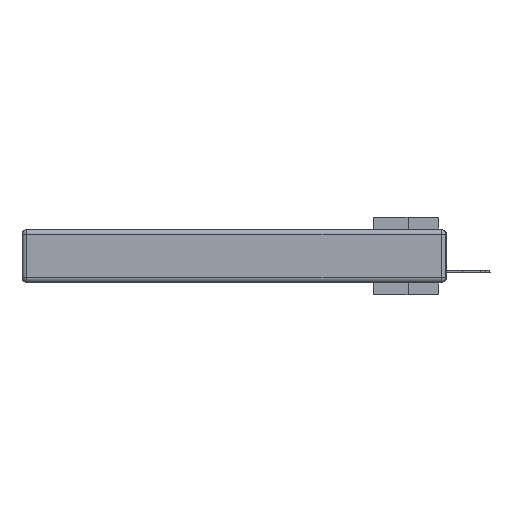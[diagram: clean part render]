
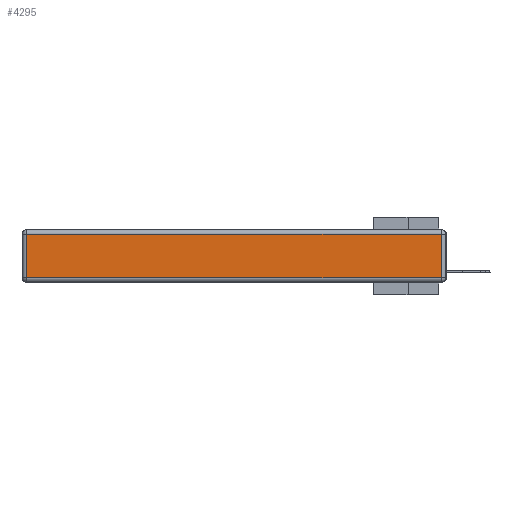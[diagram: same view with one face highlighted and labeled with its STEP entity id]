
A CAD part, left-side view. The second image highlights one B-rep face of the part: STEP entity #4295.
In plain terms, the highlighted planar face has unit normal (-1, 0, 0).
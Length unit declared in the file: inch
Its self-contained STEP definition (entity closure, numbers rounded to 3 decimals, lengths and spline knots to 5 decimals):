
#3373 = VECTOR ( 'NONE', #16008, 39.37008 ) ;
#3654 = VERTEX_POINT ( 'NONE', #3738 ) ;
#3738 = CARTESIAN_POINT ( 'NONE',  ( 0., 0.03, -0.03 ) ) ;
#4295 = ADVANCED_FACE ( 'NONE', ( #15948 ), #12384, .T. ) ;
#4736 = LINE ( 'NONE', #27565, #24641 ) ;
#5102 = ORIENTED_EDGE ( 'NONE', *, *, #26603, .T. ) ;
#5392 = CARTESIAN_POINT ( 'NONE',  ( 0., 2.72, -0.343 ) ) ;
#5779 = CARTESIAN_POINT ( 'NONE',  ( 0., 0., -0.313 ) ) ;
#5972 = DIRECTION ( 'NONE',  ( -1., 0., 0. ) ) ;
#6098 = VECTOR ( 'NONE', #14090, 39.37008 ) ;
#9346 = CARTESIAN_POINT ( 'NONE',  ( 0., 0.03, -0.313 ) ) ;
#10576 = VERTEX_POINT ( 'NONE', #12499 ) ;
#10674 = LINE ( 'NONE', #5779, #11025 ) ;
#11025 = VECTOR ( 'NONE', #21123, 39.37008 ) ;
#12384 = PLANE ( 'NONE',  #12468 ) ;
#12468 = AXIS2_PLACEMENT_3D ( 'NONE', #19115, #5972, #16828 ) ;
#12499 = CARTESIAN_POINT ( 'NONE',  ( 0., 2.72, -0.313 ) ) ;
#13677 = CARTESIAN_POINT ( 'NONE',  ( 0., 0.03, -0.343 ) ) ;
#14090 = DIRECTION ( 'NONE',  ( 0., 0., -1. ) ) ;
#14199 = ORIENTED_EDGE ( 'NONE', *, *, #22095, .T. ) ;
#15948 = FACE_OUTER_BOUND ( 'NONE', #21236, .T. ) ;
#16008 = DIRECTION ( 'NONE',  ( 0., 0., 1. ) ) ;
#16828 = DIRECTION ( 'NONE',  ( 0., 0., 1. ) ) ;
#19011 = DIRECTION ( 'NONE',  ( 0., 1., 0. ) ) ;
#19115 = CARTESIAN_POINT ( 'NONE',  ( 0., 0., -0.343 ) ) ;
#19346 = VERTEX_POINT ( 'NONE', #9346 ) ;
#21123 = DIRECTION ( 'NONE',  ( 0., -1., 0. ) ) ;
#21236 = EDGE_LOOP ( 'NONE', ( #14199, #5102, #22889, #23005 ) ) ;
#21786 = CARTESIAN_POINT ( 'NONE',  ( 0., 2.72, -0.03 ) ) ;
#21869 = LINE ( 'NONE', #13677, #3373 ) ;
#22095 = EDGE_CURVE ( 'NONE', #10576, #19346, #10674, .T. ) ;
#22889 = ORIENTED_EDGE ( 'NONE', *, *, #23967, .T. ) ;
#23005 = ORIENTED_EDGE ( 'NONE', *, *, #23914, .T. ) ;
#23914 = EDGE_CURVE ( 'NONE', #24633, #10576, #25692, .T. ) ;
#23967 = EDGE_CURVE ( 'NONE', #3654, #24633, #4736, .T. ) ;
#24633 = VERTEX_POINT ( 'NONE', #21786 ) ;
#24641 = VECTOR ( 'NONE', #19011, 39.37008 ) ;
#25692 = LINE ( 'NONE', #5392, #6098 ) ;
#26603 = EDGE_CURVE ( 'NONE', #19346, #3654, #21869, .T. ) ;
#27565 = CARTESIAN_POINT ( 'NONE',  ( 0., 2.75, -0.03 ) ) ;
